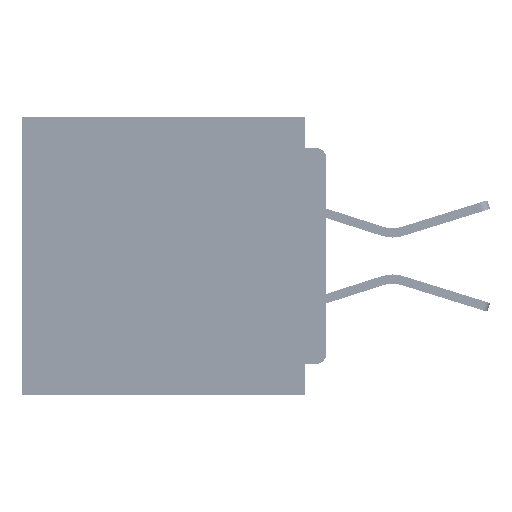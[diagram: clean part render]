
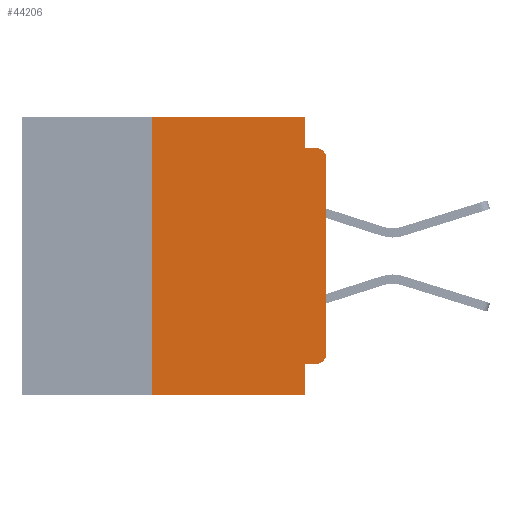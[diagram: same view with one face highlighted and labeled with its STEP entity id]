
A CAD part, left-side view. The second image highlights one B-rep face of the part: STEP entity #44206.
In plain terms, the highlighted planar face has unit normal (-1, 0, 0).
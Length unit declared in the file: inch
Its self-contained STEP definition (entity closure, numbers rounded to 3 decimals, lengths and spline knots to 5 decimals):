
#389 = VERTEX_POINT ( 'NONE', #56349 ) ;
#1810 = CARTESIAN_POINT ( 'NONE',  ( 0., 0.25, -0.4 ) ) ;
#1901 = LINE ( 'NONE', #2886, #41802 ) ;
#2146 = CARTESIAN_POINT ( 'NONE',  ( 0., 0.031, -0.355 ) ) ;
#2424 = CIRCLE ( 'NONE', #35348, 0.015 ) ;
#2464 = EDGE_CURVE ( 'NONE', #389, #22081, #2424, .T. ) ;
#2886 = CARTESIAN_POINT ( 'NONE',  ( 0., 0.437, 0. ) ) ;
#3582 = EDGE_CURVE ( 'NONE', #12946, #7138, #39673, .T. ) ;
#3596 = ORIENTED_EDGE ( 'NONE', *, *, #3882, .F. ) ;
#3882 = EDGE_CURVE ( 'NONE', #12946, #48624, #33971, .T. ) ;
#4192 = EDGE_CURVE ( 'NONE', #52691, #22081, #31135, .T. ) ;
#4512 = DIRECTION ( 'NONE',  ( 0., 0., -1. ) ) ;
#4711 = DIRECTION ( 'NONE',  ( 0., 0., -1. ) ) ;
#6019 = CARTESIAN_POINT ( 'NONE',  ( 0., 0.031, -0.045 ) ) ;
#6512 = CARTESIAN_POINT ( 'NONE',  ( 0., 0.031, 0. ) ) ;
#7138 = VERTEX_POINT ( 'NONE', #48030 ) ;
#7300 = VECTOR ( 'NONE', #4711, 39.37008 ) ;
#9222 = AXIS2_PLACEMENT_3D ( 'NONE', #33837, #49576, #18371 ) ;
#11755 = DIRECTION ( 'NONE',  ( 0., 0., -1. ) ) ;
#12946 = VERTEX_POINT ( 'NONE', #18306 ) ;
#13115 = PLANE ( 'NONE',  #9222 ) ;
#13121 = CARTESIAN_POINT ( 'NONE',  ( 0., 0., -0.355 ) ) ;
#13440 = VECTOR ( 'NONE', #20076, 39.37008 ) ;
#13802 = DIRECTION ( 'NONE',  ( 0., 0., 1. ) ) ;
#16161 = ORIENTED_EDGE ( 'NONE', *, *, #2464, .T. ) ;
#16346 = ORIENTED_EDGE ( 'NONE', *, *, #3582, .T. ) ;
#16635 = VECTOR ( 'NONE', #38501, 39.37008 ) ;
#17089 = DIRECTION ( 'NONE',  ( 0., 0., -1. ) ) ;
#17150 = DIRECTION ( 'NONE',  ( -1., 0., 0. ) ) ;
#17230 = CARTESIAN_POINT ( 'NONE',  ( 0., 0.015, -0.06 ) ) ;
#17296 = VECTOR ( 'NONE', #67540, 39.37008 ) ;
#18306 = CARTESIAN_POINT ( 'NONE',  ( 0., 0.015, -0.355 ) ) ;
#18371 = DIRECTION ( 'NONE',  ( 0., 0., -1. ) ) ;
#18403 = ORIENTED_EDGE ( 'NONE', *, *, #21946, .F. ) ;
#20076 = DIRECTION ( 'NONE',  ( 0., -1., 0. ) ) ;
#20130 = VECTOR ( 'NONE', #23553, 39.37008 ) ;
#21123 = LINE ( 'NONE', #67128, #7300 ) ;
#21946 = EDGE_CURVE ( 'NONE', #48624, #40725, #21123, .T. ) ;
#22081 = VERTEX_POINT ( 'NONE', #26751 ) ;
#23368 = VECTOR ( 'NONE', #11755, 39.37008 ) ;
#23553 = DIRECTION ( 'NONE',  ( 0., 1., 0. ) ) ;
#26013 = LINE ( 'NONE', #6512, #23368 ) ;
#26751 = CARTESIAN_POINT ( 'NONE',  ( 0., 0.015, -0.045 ) ) ;
#28903 = LINE ( 'NONE', #30285, #13440 ) ;
#28948 = LINE ( 'NONE', #29034, #39510 ) ;
#29034 = CARTESIAN_POINT ( 'NONE',  ( 0., 0.25, -0.4 ) ) ;
#29058 = ORIENTED_EDGE ( 'NONE', *, *, #29365, .F. ) ;
#29365 = EDGE_CURVE ( 'NONE', #41409, #30218, #28948, .T. ) ;
#30218 = VERTEX_POINT ( 'NONE', #52194 ) ;
#30285 = CARTESIAN_POINT ( 'NONE',  ( 0., 0.437, -0.4 ) ) ;
#31135 = LINE ( 'NONE', #62303, #17296 ) ;
#32634 = EDGE_CURVE ( 'NONE', #32969, #52691, #26013, .T. ) ;
#32969 = VERTEX_POINT ( 'NONE', #40127 ) ;
#33298 = CARTESIAN_POINT ( 'NONE',  ( 0., 0., 0. ) ) ;
#33837 = CARTESIAN_POINT ( 'NONE',  ( 0., 0.437, 0. ) ) ;
#33971 = LINE ( 'NONE', #13121, #20130 ) ;
#35343 = EDGE_LOOP ( 'NONE', ( #57793, #16161, #57335, #36404, #56400, #29058, #54486, #18403, #3596, #16346 ) ) ;
#35348 = AXIS2_PLACEMENT_3D ( 'NONE', #17230, #17150, #17089 ) ;
#35685 = DIRECTION ( 'NONE',  ( -1., 0., 0. ) ) ;
#36404 = ORIENTED_EDGE ( 'NONE', *, *, #32634, .F. ) ;
#38501 = DIRECTION ( 'NONE',  ( 0., 0., 1. ) ) ;
#39246 = DIRECTION ( 'NONE',  ( 0., -1., 0. ) ) ;
#39510 = VECTOR ( 'NONE', #13802, 39.37008 ) ;
#39673 = CIRCLE ( 'NONE', #40605, 0.015 ) ;
#40127 = CARTESIAN_POINT ( 'NONE',  ( 0., 0.031, 0. ) ) ;
#40605 = AXIS2_PLACEMENT_3D ( 'NONE', #66921, #35685, #4512 ) ;
#40725 = VERTEX_POINT ( 'NONE', #42178 ) ;
#41409 = VERTEX_POINT ( 'NONE', #1810 ) ;
#41802 = VECTOR ( 'NONE', #39246, 39.37008 ) ;
#42178 = CARTESIAN_POINT ( 'NONE',  ( 0., 0.031, -0.4 ) ) ;
#44206 = ADVANCED_FACE ( 'NONE', ( #47385 ), #13115, .F. ) ;
#47385 = FACE_OUTER_BOUND ( 'NONE', #35343, .T. ) ;
#48030 = CARTESIAN_POINT ( 'NONE',  ( 0., 0., -0.34 ) ) ;
#48624 = VERTEX_POINT ( 'NONE', #2146 ) ;
#49247 = EDGE_CURVE ( 'NONE', #30218, #32969, #1901, .T. ) ;
#49576 = DIRECTION ( 'NONE',  ( 1., 0., 0. ) ) ;
#52194 = CARTESIAN_POINT ( 'NONE',  ( 0., 0.25, 0. ) ) ;
#52691 = VERTEX_POINT ( 'NONE', #6019 ) ;
#52850 = EDGE_CURVE ( 'NONE', #7138, #389, #58183, .T. ) ;
#53125 = EDGE_CURVE ( 'NONE', #41409, #40725, #28903, .T. ) ;
#54486 = ORIENTED_EDGE ( 'NONE', *, *, #53125, .T. ) ;
#56349 = CARTESIAN_POINT ( 'NONE',  ( 0., 0., -0.06 ) ) ;
#56400 = ORIENTED_EDGE ( 'NONE', *, *, #49247, .F. ) ;
#57335 = ORIENTED_EDGE ( 'NONE', *, *, #4192, .F. ) ;
#57793 = ORIENTED_EDGE ( 'NONE', *, *, #52850, .T. ) ;
#58183 = LINE ( 'NONE', #33298, #16635 ) ;
#62303 = CARTESIAN_POINT ( 'NONE',  ( 0., 0., -0.045 ) ) ;
#66921 = CARTESIAN_POINT ( 'NONE',  ( 0., 0.015, -0.34 ) ) ;
#67128 = CARTESIAN_POINT ( 'NONE',  ( 0., 0.031, -0.4 ) ) ;
#67540 = DIRECTION ( 'NONE',  ( 0., -1., 0. ) ) ;
